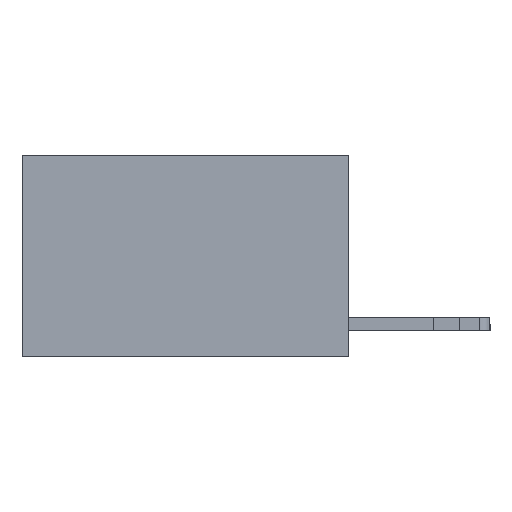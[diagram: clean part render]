
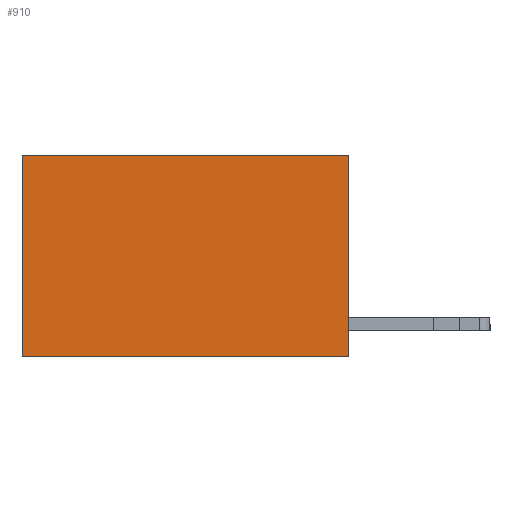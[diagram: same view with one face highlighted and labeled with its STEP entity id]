
A CAD part, left-side view. The second image highlights one B-rep face of the part: STEP entity #910.
In plain terms, the highlighted planar face has unit normal (-1, 0, 0).
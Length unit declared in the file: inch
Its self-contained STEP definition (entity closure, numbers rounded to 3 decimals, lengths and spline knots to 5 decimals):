
#910 = ADVANCED_FACE ( 'NONE', ( #17877 ), #2976, .F. ) ;
#1549 = DIRECTION ( 'NONE',  ( 0., 0., -1. ) ) ;
#1926 = EDGE_CURVE ( 'NONE', #19485, #7469, #18155, .T. ) ;
#2976 = PLANE ( 'NONE',  #7790 ) ;
#2989 = DIRECTION ( 'NONE',  ( 0., 1., 0. ) ) ;
#3136 = CARTESIAN_POINT ( 'NONE',  ( 0.2625, 0.6, -0.37 ) ) ;
#3990 = CARTESIAN_POINT ( 'NONE',  ( 0.2625, 0.6, 0. ) ) ;
#4411 = CARTESIAN_POINT ( 'NONE',  ( 0.2625, 0., 0. ) ) ;
#4468 = EDGE_CURVE ( 'NONE', #16646, #7469, #17965, .T. ) ;
#5810 = VECTOR ( 'NONE', #13404, 39.37008 ) ;
#6820 = VERTEX_POINT ( 'NONE', #9224 ) ;
#7469 = VERTEX_POINT ( 'NONE', #3136 ) ;
#7790 = AXIS2_PLACEMENT_3D ( 'NONE', #13121, #14642, #19601 ) ;
#7814 = EDGE_CURVE ( 'NONE', #6820, #19485, #8038, .T. ) ;
#8038 = LINE ( 'NONE', #20906, #20067 ) ;
#8056 = LINE ( 'NONE', #4411, #17184 ) ;
#8906 = VECTOR ( 'NONE', #1549, 39.37008 ) ;
#9224 = CARTESIAN_POINT ( 'NONE',  ( 0.2625, 0., 0. ) ) ;
#9459 = DIRECTION ( 'NONE',  ( 0., 0., -1. ) ) ;
#11594 = CARTESIAN_POINT ( 'NONE',  ( 0.2625, 0.6, 0. ) ) ;
#13121 = CARTESIAN_POINT ( 'NONE',  ( 0.2625, 0., 0. ) ) ;
#13404 = DIRECTION ( 'NONE',  ( 0., 1., 0. ) ) ;
#14532 = ORIENTED_EDGE ( 'NONE', *, *, #1926, .F. ) ;
#14642 = DIRECTION ( 'NONE',  ( 1., 0., 0. ) ) ;
#16134 = ORIENTED_EDGE ( 'NONE', *, *, #16716, .T. ) ;
#16646 = VERTEX_POINT ( 'NONE', #3990 ) ;
#16716 = EDGE_CURVE ( 'NONE', #6820, #16646, #8056, .T. ) ;
#16907 = ORIENTED_EDGE ( 'NONE', *, *, #7814, .F. ) ;
#17184 = VECTOR ( 'NONE', #2989, 39.37008 ) ;
#17466 = ORIENTED_EDGE ( 'NONE', *, *, #4468, .T. ) ;
#17877 = FACE_OUTER_BOUND ( 'NONE', #19479, .T. ) ;
#17965 = LINE ( 'NONE', #11594, #8906 ) ;
#18155 = LINE ( 'NONE', #19988, #5810 ) ;
#18359 = CARTESIAN_POINT ( 'NONE',  ( 0.2625, 0., -0.37 ) ) ;
#19479 = EDGE_LOOP ( 'NONE', ( #17466, #14532, #16907, #16134 ) ) ;
#19485 = VERTEX_POINT ( 'NONE', #18359 ) ;
#19601 = DIRECTION ( 'NONE',  ( 0., 0., -1. ) ) ;
#19988 = CARTESIAN_POINT ( 'NONE',  ( 0.2625, 0., -0.37 ) ) ;
#20067 = VECTOR ( 'NONE', #9459, 39.37008 ) ;
#20906 = CARTESIAN_POINT ( 'NONE',  ( 0.2625, 0., 0. ) ) ;
